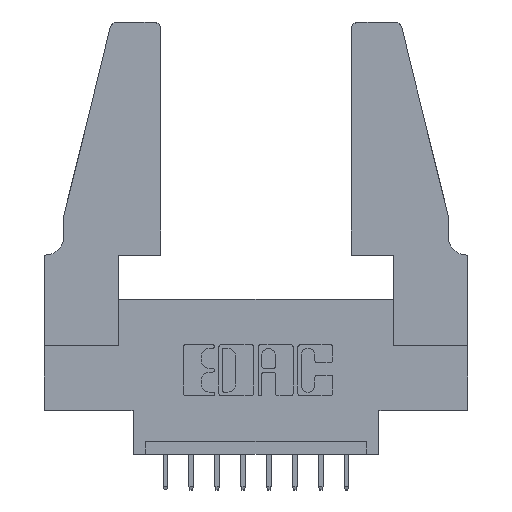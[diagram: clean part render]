
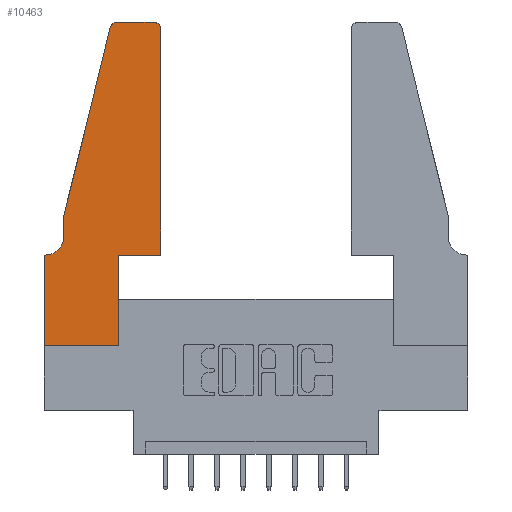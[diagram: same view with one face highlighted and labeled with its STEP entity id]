
A CAD part, top view. The second image highlights one B-rep face of the part: STEP entity #10463.
In plain terms, the highlighted planar face has unit normal (0, 0, 1).
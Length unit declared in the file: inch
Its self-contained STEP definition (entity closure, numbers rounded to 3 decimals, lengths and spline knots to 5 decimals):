
#277 = EDGE_CURVE ( 'NONE', #10353, #11289, #7788, .T. ) ;
#589 = EDGE_CURVE ( 'NONE', #3418, #9237, #9635, .T. ) ;
#946 = ORIENTED_EDGE ( 'NONE', *, *, #6639, .T. ) ;
#1104 = DIRECTION ( 'NONE',  ( 1., 0., 0. ) ) ;
#1224 = DIRECTION ( 'NONE',  ( 1., 0., 0. ) ) ;
#1487 = CARTESIAN_POINT ( 'NONE',  ( 0.0755, 0.5, 0.37 ) ) ;
#1537 = VERTEX_POINT ( 'NONE', #11331 ) ;
#1547 = CARTESIAN_POINT ( 'NONE',  ( 0., 0., 0.37 ) ) ;
#1678 = CARTESIAN_POINT ( 'NONE',  ( 0.4205, 1.22, 0.37 ) ) ;
#1714 = DIRECTION ( 'NONE',  ( 1., 0., 0. ) ) ;
#1934 = ORIENTED_EDGE ( 'NONE', *, *, #2448, .T. ) ;
#1953 = PLANE ( 'NONE',  #7311 ) ;
#2052 = CARTESIAN_POINT ( 'NONE',  ( 0.0055, 0.42, 0.37 ) ) ;
#2107 = EDGE_CURVE ( 'NONE', #9987, #1537, #6788, .T. ) ;
#2114 = CARTESIAN_POINT ( 'NONE',  ( 0.0755, 0.5, 0.37 ) ) ;
#2117 = DIRECTION ( 'NONE',  ( -1., 0., 0. ) ) ;
#2299 = EDGE_CURVE ( 'NONE', #9482, #9562, #9098, .T. ) ;
#2306 = VECTOR ( 'NONE', #2674, 39.37008 ) ;
#2407 = LINE ( 'NONE', #1547, #10226 ) ;
#2448 = EDGE_CURVE ( 'NONE', #9018, #3418, #9481, .T. ) ;
#2607 = CIRCLE ( 'NONE', #7058, 0.03 ) ;
#2674 = DIRECTION ( 'NONE',  ( 1., 0., 0. ) ) ;
#2709 = CARTESIAN_POINT ( 'NONE',  ( 0.4505, 1.22, 0.37 ) ) ;
#2849 = ORIENTED_EDGE ( 'NONE', *, *, #8968, .T. ) ;
#2922 = VERTEX_POINT ( 'NONE', #9209 ) ;
#3182 = CIRCLE ( 'NONE', #4854, 0.03 ) ;
#3185 = CARTESIAN_POINT ( 'NONE',  ( 0., 0., 0.37 ) ) ;
#3418 = VERTEX_POINT ( 'NONE', #6961 ) ;
#3455 = CARTESIAN_POINT ( 'NONE',  ( 0.2865, 0.35, 0.37 ) ) ;
#3835 = CARTESIAN_POINT ( 'NONE',  ( 0., 0.35, 0.37 ) ) ;
#3912 = VERTEX_POINT ( 'NONE', #9431 ) ;
#4162 = EDGE_CURVE ( 'NONE', #6422, #9482, #3182, .T. ) ;
#4405 = VECTOR ( 'NONE', #1224, 39.37008 ) ;
#4466 = CARTESIAN_POINT ( 'NONE',  ( 0.4505, 0.35, 0.37 ) ) ;
#4492 = CARTESIAN_POINT ( 'NONE',  ( 0.2605, 1.25, 0.37 ) ) ;
#4629 = DIRECTION ( 'NONE',  ( 0., -1., 0. ) ) ;
#4770 = ORIENTED_EDGE ( 'NONE', *, *, #7466, .T. ) ;
#4854 = AXIS2_PLACEMENT_3D ( 'NONE', #7650, #6726, #1714 ) ;
#5016 = CARTESIAN_POINT ( 'NONE',  ( 0.0055, 0.35, 0.37 ) ) ;
#5442 = ORIENTED_EDGE ( 'NONE', *, *, #8685, .T. ) ;
#5715 = CARTESIAN_POINT ( 'NONE',  ( 0.284, 1.25, 0.37 ) ) ;
#5739 = EDGE_CURVE ( 'NONE', #2922, #10353, #12352, .T. ) ;
#5758 = ORIENTED_EDGE ( 'NONE', *, *, #277, .T. ) ;
#5956 = CARTESIAN_POINT ( 'NONE',  ( 0., 0.35, 0.37 ) ) ;
#6422 = VERTEX_POINT ( 'NONE', #5715 ) ;
#6639 = EDGE_CURVE ( 'NONE', #11289, #9987, #2407, .T. ) ;
#6726 = DIRECTION ( 'NONE',  ( 0., 0., 1. ) ) ;
#6788 = LINE ( 'NONE', #9813, #2306 ) ;
#6854 = CARTESIAN_POINT ( 'NONE',  ( 0.2865, 0.35, 0.37 ) ) ;
#6890 = ORIENTED_EDGE ( 'NONE', *, *, #5739, .T. ) ;
#6961 = CARTESIAN_POINT ( 'NONE',  ( 0.4505, 0.35, 0.37 ) ) ;
#7058 = AXIS2_PLACEMENT_3D ( 'NONE', #1678, #7875, #12739 ) ;
#7067 = EDGE_LOOP ( 'NONE', ( #5442, #12318, #7161, #2849, #6890, #5758, #946, #10651, #10755, #1934, #9952, #4770 ) ) ;
#7161 = ORIENTED_EDGE ( 'NONE', *, *, #2299, .T. ) ;
#7311 = AXIS2_PLACEMENT_3D ( 'NONE', #5956, #10004, #1104 ) ;
#7456 = DIRECTION ( 'NONE',  ( 0., 1., 0. ) ) ;
#7466 = EDGE_CURVE ( 'NONE', #9237, #3912, #2607, .T. ) ;
#7650 = CARTESIAN_POINT ( 'NONE',  ( 0.284, 1.22, 0.37 ) ) ;
#7769 = DIRECTION ( 'NONE',  ( 0., 1., 0. ) ) ;
#7788 = LINE ( 'NONE', #11801, #8229 ) ;
#7875 = DIRECTION ( 'NONE',  ( 0., 0., 1. ) ) ;
#8004 = VECTOR ( 'NONE', #7456, 39.37008 ) ;
#8193 = DIRECTION ( 'NONE',  ( 0., -1., 0. ) ) ;
#8229 = VECTOR ( 'NONE', #11864, 39.37008 ) ;
#8234 = CARTESIAN_POINT ( 'NONE',  ( 0.4505, 0.35, 0.37 ) ) ;
#8299 = EDGE_CURVE ( 'NONE', #1537, #9018, #8695, .T. ) ;
#8300 = CARTESIAN_POINT ( 'NONE',  ( 0.25487, 1.22718, 0.37 ) ) ;
#8685 = EDGE_CURVE ( 'NONE', #3912, #6422, #12412, .T. ) ;
#8695 = LINE ( 'NONE', #6854, #8963 ) ;
#8957 = CARTESIAN_POINT ( 'NONE',  ( 0.0755, 0.5, 0.37 ) ) ;
#8963 = VECTOR ( 'NONE', #7769, 39.37008 ) ;
#8968 = EDGE_CURVE ( 'NONE', #9562, #2922, #11156, .T. ) ;
#9018 = VERTEX_POINT ( 'NONE', #3455 ) ;
#9098 = LINE ( 'NONE', #8957, #11785 ) ;
#9209 = CARTESIAN_POINT ( 'NONE',  ( 0.0755, 0.42, 0.37 ) ) ;
#9228 = AXIS2_PLACEMENT_3D ( 'NONE', #2052, #11224, #2117 ) ;
#9237 = VERTEX_POINT ( 'NONE', #2709 ) ;
#9431 = CARTESIAN_POINT ( 'NONE',  ( 0.4205, 1.25, 0.37 ) ) ;
#9481 = LINE ( 'NONE', #8234, #4405 ) ;
#9482 = VERTEX_POINT ( 'NONE', #8300 ) ;
#9562 = VERTEX_POINT ( 'NONE', #1487 ) ;
#9635 = LINE ( 'NONE', #4466, #8004 ) ;
#9813 = CARTESIAN_POINT ( 'NONE',  ( 0., 0., 0.37 ) ) ;
#9937 = FACE_OUTER_BOUND ( 'NONE', #7067, .T. ) ;
#9952 = ORIENTED_EDGE ( 'NONE', *, *, #589, .T. ) ;
#9987 = VERTEX_POINT ( 'NONE', #3185 ) ;
#10004 = DIRECTION ( 'NONE',  ( 0., 0., 1. ) ) ;
#10161 = DIRECTION ( 'NONE',  ( -0.239, -0.971, 0. ) ) ;
#10226 = VECTOR ( 'NONE', #4629, 39.37008 ) ;
#10353 = VERTEX_POINT ( 'NONE', #5016 ) ;
#10404 = DIRECTION ( 'NONE',  ( -1., 0., 0. ) ) ;
#10463 = ADVANCED_FACE ( 'NONE', ( #9937 ), #1953, .T. ) ;
#10651 = ORIENTED_EDGE ( 'NONE', *, *, #2107, .T. ) ;
#10755 = ORIENTED_EDGE ( 'NONE', *, *, #8299, .T. ) ;
#10882 = VECTOR ( 'NONE', #10404, 39.37008 ) ;
#11156 = LINE ( 'NONE', #2114, #11506 ) ;
#11224 = DIRECTION ( 'NONE',  ( 0., 0., -1. ) ) ;
#11289 = VERTEX_POINT ( 'NONE', #3835 ) ;
#11331 = CARTESIAN_POINT ( 'NONE',  ( 0.2865, 0., 0.37 ) ) ;
#11506 = VECTOR ( 'NONE', #8193, 39.37008 ) ;
#11785 = VECTOR ( 'NONE', #10161, 39.37008 ) ;
#11801 = CARTESIAN_POINT ( 'NONE',  ( 0.0755, 0.35, 0.37 ) ) ;
#11864 = DIRECTION ( 'NONE',  ( -1., 0., 0. ) ) ;
#12318 = ORIENTED_EDGE ( 'NONE', *, *, #4162, .T. ) ;
#12352 = CIRCLE ( 'NONE', #9228, 0.07 ) ;
#12412 = LINE ( 'NONE', #4492, #10882 ) ;
#12739 = DIRECTION ( 'NONE',  ( 1., 0., 0. ) ) ;
